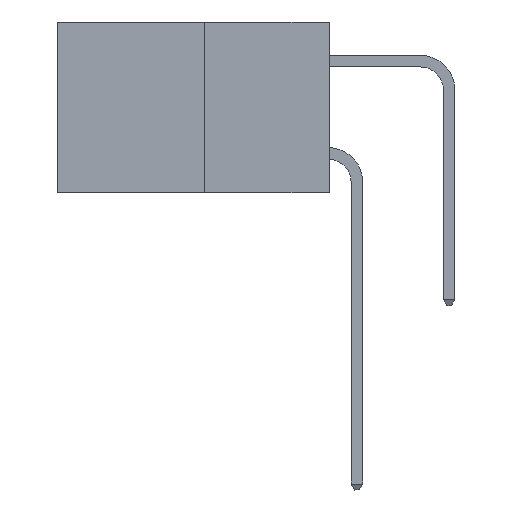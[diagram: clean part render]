
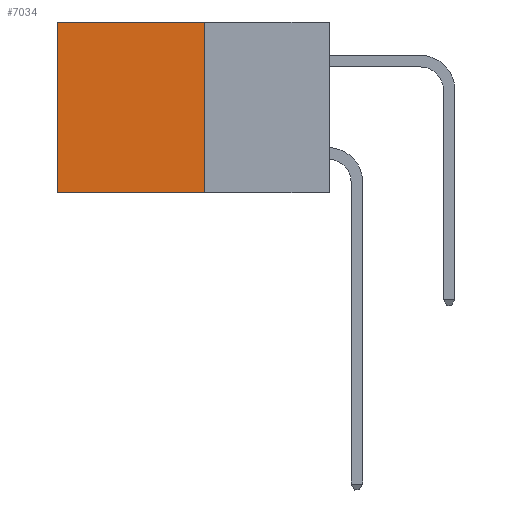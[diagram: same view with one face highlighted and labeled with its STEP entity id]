
A CAD part, left-side view. The second image highlights one B-rep face of the part: STEP entity #7034.
In plain terms, the highlighted planar face has unit normal (-1, 0, 0).
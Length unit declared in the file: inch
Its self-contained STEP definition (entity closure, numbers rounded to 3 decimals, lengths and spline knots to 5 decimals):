
#392 = LINE ( 'NONE', #4052, #20742 ) ;
#683 = EDGE_CURVE ( 'NONE', #7513, #4707, #11965, .T. ) ;
#2087 = EDGE_CURVE ( 'NONE', #5289, #4707, #15380, .T. ) ;
#2153 = EDGE_LOOP ( 'NONE', ( #14810, #26179, #4822, #20615 ) ) ;
#4052 = CARTESIAN_POINT ( 'NONE',  ( 0.277, 0.27, 0. ) ) ;
#4298 = DIRECTION ( 'NONE',  ( 0., 0., -1. ) ) ;
#4707 = VERTEX_POINT ( 'NONE', #26278 ) ;
#4822 = ORIENTED_EDGE ( 'NONE', *, *, #21572, .F. ) ;
#5289 = VERTEX_POINT ( 'NONE', #6191 ) ;
#6142 = AXIS2_PLACEMENT_3D ( 'NONE', #6961, #19244, #7051 ) ;
#6191 = CARTESIAN_POINT ( 'NONE',  ( 0.277, 0.59, 0. ) ) ;
#6961 = CARTESIAN_POINT ( 'NONE',  ( 0.277, 0.27, -0.37 ) ) ;
#7034 = ADVANCED_FACE ( 'NONE', ( #9541 ), #17179, .F. ) ;
#7051 = DIRECTION ( 'NONE',  ( 0., 0., -1. ) ) ;
#7334 = DIRECTION ( 'NONE',  ( 0., 1., 0. ) ) ;
#7513 = VERTEX_POINT ( 'NONE', #16554 ) ;
#7828 = VECTOR ( 'NONE', #13338, 39.37008 ) ;
#8790 = VECTOR ( 'NONE', #4298, 39.37008 ) ;
#9541 = FACE_OUTER_BOUND ( 'NONE', #2153, .T. ) ;
#9994 = VECTOR ( 'NONE', #11236, 39.37008 ) ;
#11236 = DIRECTION ( 'NONE',  ( 0., 0., -1. ) ) ;
#11531 = CARTESIAN_POINT ( 'NONE',  ( 0.277, 0.59, -0.37 ) ) ;
#11965 = LINE ( 'NONE', #19121, #7828 ) ;
#13338 = DIRECTION ( 'NONE',  ( 0., 1., 0. ) ) ;
#14214 = LINE ( 'NONE', #22512, #8790 ) ;
#14810 = ORIENTED_EDGE ( 'NONE', *, *, #2087, .T. ) ;
#15380 = LINE ( 'NONE', #11531, #9994 ) ;
#16554 = CARTESIAN_POINT ( 'NONE',  ( 0.277, 0.27, -0.37 ) ) ;
#17179 = PLANE ( 'NONE',  #6142 ) ;
#19121 = CARTESIAN_POINT ( 'NONE',  ( 0.277, 0.27, -0.37 ) ) ;
#19225 = CARTESIAN_POINT ( 'NONE',  ( 0.277, 0.27, 0. ) ) ;
#19244 = DIRECTION ( 'NONE',  ( 1., 0., 0. ) ) ;
#20615 = ORIENTED_EDGE ( 'NONE', *, *, #24843, .T. ) ;
#20742 = VECTOR ( 'NONE', #7334, 39.37008 ) ;
#21572 = EDGE_CURVE ( 'NONE', #23879, #7513, #14214, .T. ) ;
#22512 = CARTESIAN_POINT ( 'NONE',  ( 0.277, 0.27, -0.37 ) ) ;
#23879 = VERTEX_POINT ( 'NONE', #19225 ) ;
#24843 = EDGE_CURVE ( 'NONE', #23879, #5289, #392, .T. ) ;
#26179 = ORIENTED_EDGE ( 'NONE', *, *, #683, .F. ) ;
#26278 = CARTESIAN_POINT ( 'NONE',  ( 0.277, 0.59, -0.37 ) ) ;
